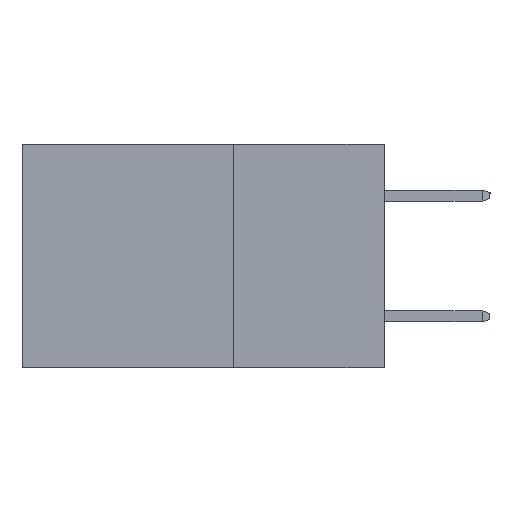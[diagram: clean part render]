
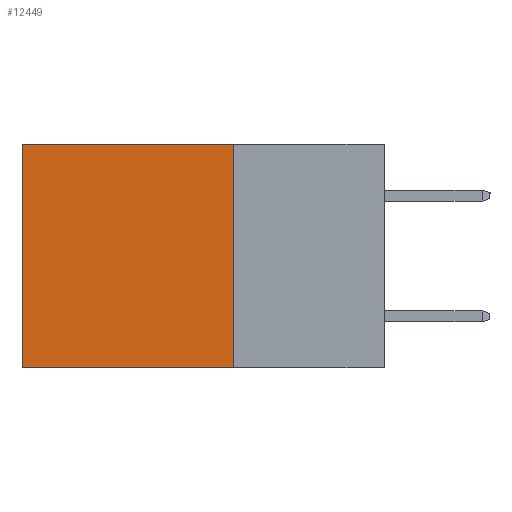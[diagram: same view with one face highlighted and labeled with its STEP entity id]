
A CAD part, left-side view. The second image highlights one B-rep face of the part: STEP entity #12449.
In plain terms, the highlighted planar face has unit normal (-1, 0, 0).
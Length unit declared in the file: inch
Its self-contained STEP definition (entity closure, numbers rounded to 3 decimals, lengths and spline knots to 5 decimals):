
#1749 = EDGE_CURVE ( 'NONE', #22616, #8248, #22161, .T. ) ;
#2102 = ORIENTED_EDGE ( 'NONE', *, *, #2652, .T. ) ;
#2652 = EDGE_CURVE ( 'NONE', #8248, #11855, #10612, .T. ) ;
#2736 = CARTESIAN_POINT ( 'NONE',  ( 0.2615, 0.25, 0. ) ) ;
#3656 = DIRECTION ( 'NONE',  ( 0., 0., -1. ) ) ;
#3785 = CARTESIAN_POINT ( 'NONE',  ( 0.2615, 0.6, 0. ) ) ;
#4331 = EDGE_CURVE ( 'NONE', #11485, #11855, #14083, .T. ) ;
#4356 = DIRECTION ( 'NONE',  ( 0., 1., 0. ) ) ;
#4534 = DIRECTION ( 'NONE',  ( 0., 1., 0. ) ) ;
#6663 = CARTESIAN_POINT ( 'NONE',  ( 0.2615, 0.6, -0.37 ) ) ;
#7098 = LINE ( 'NONE', #14901, #22535 ) ;
#7576 = CARTESIAN_POINT ( 'NONE',  ( 0.2615, 0.25, 0. ) ) ;
#8248 = VERTEX_POINT ( 'NONE', #3785 ) ;
#8343 = VECTOR ( 'NONE', #18041, 39.37008 ) ;
#9282 = PLANE ( 'NONE',  #12033 ) ;
#9837 = EDGE_CURVE ( 'NONE', #22616, #11485, #7098, .T. ) ;
#10308 = ORIENTED_EDGE ( 'NONE', *, *, #4331, .F. ) ;
#10612 = LINE ( 'NONE', #20072, #8343 ) ;
#11485 = VERTEX_POINT ( 'NONE', #13087 ) ;
#11855 = VERTEX_POINT ( 'NONE', #6663 ) ;
#12033 = AXIS2_PLACEMENT_3D ( 'NONE', #12991, #20897, #3656 ) ;
#12449 = ADVANCED_FACE ( 'NONE', ( #21145 ), #9282, .F. ) ;
#12991 = CARTESIAN_POINT ( 'NONE',  ( 0.2615, 0.25, -0.37 ) ) ;
#13087 = CARTESIAN_POINT ( 'NONE',  ( 0.2615, 0.25, -0.37 ) ) ;
#13966 = CARTESIAN_POINT ( 'NONE',  ( 0.2615, 0.25, -0.37 ) ) ;
#14083 = LINE ( 'NONE', #13966, #16268 ) ;
#14901 = CARTESIAN_POINT ( 'NONE',  ( 0.2615, 0.25, -0.37 ) ) ;
#16268 = VECTOR ( 'NONE', #4356, 39.37008 ) ;
#18041 = DIRECTION ( 'NONE',  ( 0., 0., -1. ) ) ;
#18815 = ORIENTED_EDGE ( 'NONE', *, *, #9837, .F. ) ;
#18877 = DIRECTION ( 'NONE',  ( 0., 0., -1. ) ) ;
#19298 = VECTOR ( 'NONE', #4534, 39.37008 ) ;
#20072 = CARTESIAN_POINT ( 'NONE',  ( 0.2615, 0.6, -0.37 ) ) ;
#20897 = DIRECTION ( 'NONE',  ( 1., 0., 0. ) ) ;
#21145 = FACE_OUTER_BOUND ( 'NONE', #22578, .T. ) ;
#22161 = LINE ( 'NONE', #2736, #19298 ) ;
#22535 = VECTOR ( 'NONE', #18877, 39.37008 ) ;
#22578 = EDGE_LOOP ( 'NONE', ( #2102, #10308, #18815, #23008 ) ) ;
#22616 = VERTEX_POINT ( 'NONE', #7576 ) ;
#23008 = ORIENTED_EDGE ( 'NONE', *, *, #1749, .T. ) ;
